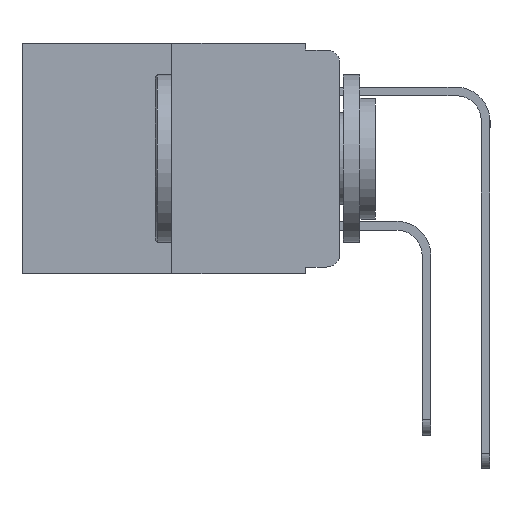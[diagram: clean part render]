
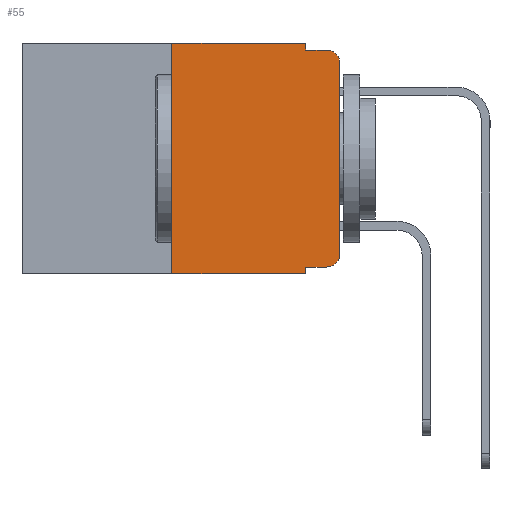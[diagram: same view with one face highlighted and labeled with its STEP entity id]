
A CAD part, left-side view. The second image highlights one B-rep face of the part: STEP entity #55.
In plain terms, the highlighted planar face has unit normal (-1, 0, 0).
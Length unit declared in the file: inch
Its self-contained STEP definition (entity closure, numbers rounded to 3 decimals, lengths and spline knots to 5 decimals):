
#55 = ADVANCED_FACE ( 'NONE', ( #3621 ), #3108, .F. ) ;
#83 = DIRECTION ( 'NONE',  ( 1., 0., 0. ) ) ;
#320 = LINE ( 'NONE', #1128, #13577 ) ;
#357 = CIRCLE ( 'NONE', #2701, 0.02 ) ;
#510 = DIRECTION ( 'NONE',  ( 0., -1., 0. ) ) ;
#694 = CARTESIAN_POINT ( 'NONE',  ( 0., 0.473, -0.343 ) ) ;
#738 = ORIENTED_EDGE ( 'NONE', *, *, #2600, .F. ) ;
#1113 = CARTESIAN_POINT ( 'NONE',  ( 0., 0.473, 0. ) ) ;
#1128 = CARTESIAN_POINT ( 'NONE',  ( 0., 0.051, 0. ) ) ;
#1188 = ORIENTED_EDGE ( 'NONE', *, *, #11584, .F. ) ;
#1362 = VECTOR ( 'NONE', #5906, 39.37008 ) ;
#1433 = VECTOR ( 'NONE', #2498, 39.37008 ) ;
#1472 = VERTEX_POINT ( 'NONE', #10219 ) ;
#1610 = ORIENTED_EDGE ( 'NONE', *, *, #7848, .F. ) ;
#1682 = EDGE_CURVE ( 'NONE', #14410, #9375, #10549, .T. ) ;
#1893 = DIRECTION ( 'NONE',  ( 0., 0., -1. ) ) ;
#2375 = CARTESIAN_POINT ( 'NONE',  ( 0., 0.051, -0.343 ) ) ;
#2498 = DIRECTION ( 'NONE',  ( 0., -1., 0. ) ) ;
#2600 = EDGE_CURVE ( 'NONE', #8962, #14410, #320, .T. ) ;
#2701 = AXIS2_PLACEMENT_3D ( 'NONE', #5745, #14416, #7051 ) ;
#3108 = PLANE ( 'NONE',  #12618 ) ;
#3146 = CARTESIAN_POINT ( 'NONE',  ( 0., 0.25, 0. ) ) ;
#3264 = CARTESIAN_POINT ( 'NONE',  ( 0., 0.051, -0.333 ) ) ;
#3621 = FACE_OUTER_BOUND ( 'NONE', #4424, .T. ) ;
#3901 = LINE ( 'NONE', #694, #16352 ) ;
#4207 = DIRECTION ( 'NONE',  ( 0., 0., 1. ) ) ;
#4424 = EDGE_LOOP ( 'NONE', ( #13570, #7392, #13951, #738, #1188, #4769, #8194, #1610, #5575, #8958 ) ) ;
#4631 = EDGE_CURVE ( 'NONE', #11760, #1472, #6729, .T. ) ;
#4769 = ORIENTED_EDGE ( 'NONE', *, *, #5276, .F. ) ;
#5276 = EDGE_CURVE ( 'NONE', #12658, #6223, #5408, .T. ) ;
#5398 = CARTESIAN_POINT ( 'NONE',  ( 0., 0.02, -0.333 ) ) ;
#5408 = LINE ( 'NONE', #3146, #12057 ) ;
#5575 = ORIENTED_EDGE ( 'NONE', *, *, #8677, .T. ) ;
#5745 = CARTESIAN_POINT ( 'NONE',  ( 0., 0.02, -0.03 ) ) ;
#5906 = DIRECTION ( 'NONE',  ( 0., 0., 1. ) ) ;
#6223 = VERTEX_POINT ( 'NONE', #9219 ) ;
#6594 = CARTESIAN_POINT ( 'NONE',  ( 0., 0., -0.03 ) ) ;
#6729 = CIRCLE ( 'NONE', #15618, 0.02 ) ;
#6971 = CARTESIAN_POINT ( 'NONE',  ( 0., 0.051, -0.01 ) ) ;
#7051 = DIRECTION ( 'NONE',  ( 0., 0., -1. ) ) ;
#7327 = LINE ( 'NONE', #8414, #10265 ) ;
#7392 = ORIENTED_EDGE ( 'NONE', *, *, #16355, .T. ) ;
#7400 = LINE ( 'NONE', #3264, #10339 ) ;
#7442 = EDGE_CURVE ( 'NONE', #12658, #9541, #3901, .T. ) ;
#7848 = EDGE_CURVE ( 'NONE', #8997, #9541, #7327, .T. ) ;
#8194 = ORIENTED_EDGE ( 'NONE', *, *, #7442, .T. ) ;
#8414 = CARTESIAN_POINT ( 'NONE',  ( 0., 0.051, 0. ) ) ;
#8677 = EDGE_CURVE ( 'NONE', #8997, #11760, #7400, .T. ) ;
#8798 = LINE ( 'NONE', #1113, #1433 ) ;
#8958 = ORIENTED_EDGE ( 'NONE', *, *, #4631, .T. ) ;
#8962 = VERTEX_POINT ( 'NONE', #9021 ) ;
#8997 = VERTEX_POINT ( 'NONE', #10331 ) ;
#9021 = CARTESIAN_POINT ( 'NONE',  ( 0., 0.051, 0. ) ) ;
#9105 = DIRECTION ( 'NONE',  ( 0., 0., -1. ) ) ;
#9219 = CARTESIAN_POINT ( 'NONE',  ( 0., 0.25, 0. ) ) ;
#9375 = VERTEX_POINT ( 'NONE', #11004 ) ;
#9541 = VERTEX_POINT ( 'NONE', #2375 ) ;
#9852 = DIRECTION ( 'NONE',  ( 0., -1., 0. ) ) ;
#10174 = VECTOR ( 'NONE', #13646, 39.37008 ) ;
#10219 = CARTESIAN_POINT ( 'NONE',  ( 0., 0., -0.313 ) ) ;
#10265 = VECTOR ( 'NONE', #1893, 39.37008 ) ;
#10331 = CARTESIAN_POINT ( 'NONE',  ( 0., 0.051, -0.333 ) ) ;
#10339 = VECTOR ( 'NONE', #510, 39.37008 ) ;
#10489 = DIRECTION ( 'NONE',  ( 0., 0., -1. ) ) ;
#10549 = LINE ( 'NONE', #6971, #10174 ) ;
#10581 = CARTESIAN_POINT ( 'NONE',  ( 0., 0.25, -0.343 ) ) ;
#10763 = VERTEX_POINT ( 'NONE', #6594 ) ;
#11004 = CARTESIAN_POINT ( 'NONE',  ( 0., 0.02, -0.01 ) ) ;
#11249 = LINE ( 'NONE', #13349, #1362 ) ;
#11584 = EDGE_CURVE ( 'NONE', #6223, #8962, #8798, .T. ) ;
#11760 = VERTEX_POINT ( 'NONE', #5398 ) ;
#11943 = DIRECTION ( 'NONE',  ( -1., 0., 0. ) ) ;
#11945 = CARTESIAN_POINT ( 'NONE',  ( 0., 0.02, -0.313 ) ) ;
#12057 = VECTOR ( 'NONE', #4207, 39.37008 ) ;
#12618 = AXIS2_PLACEMENT_3D ( 'NONE', #15040, #83, #10489 ) ;
#12658 = VERTEX_POINT ( 'NONE', #10581 ) ;
#12748 = CARTESIAN_POINT ( 'NONE',  ( 0., 0.051, -0.01 ) ) ;
#13349 = CARTESIAN_POINT ( 'NONE',  ( 0., 0., 0. ) ) ;
#13570 = ORIENTED_EDGE ( 'NONE', *, *, #13925, .T. ) ;
#13577 = VECTOR ( 'NONE', #9105, 39.37008 ) ;
#13646 = DIRECTION ( 'NONE',  ( 0., -1., 0. ) ) ;
#13925 = EDGE_CURVE ( 'NONE', #1472, #10763, #11249, .T. ) ;
#13951 = ORIENTED_EDGE ( 'NONE', *, *, #1682, .F. ) ;
#14333 = DIRECTION ( 'NONE',  ( 0., 0., -1. ) ) ;
#14410 = VERTEX_POINT ( 'NONE', #12748 ) ;
#14416 = DIRECTION ( 'NONE',  ( -1., 0., 0. ) ) ;
#15040 = CARTESIAN_POINT ( 'NONE',  ( 0., 0.473, 0. ) ) ;
#15618 = AXIS2_PLACEMENT_3D ( 'NONE', #11945, #11943, #14333 ) ;
#16352 = VECTOR ( 'NONE', #9852, 39.37008 ) ;
#16355 = EDGE_CURVE ( 'NONE', #10763, #9375, #357, .T. ) ;
